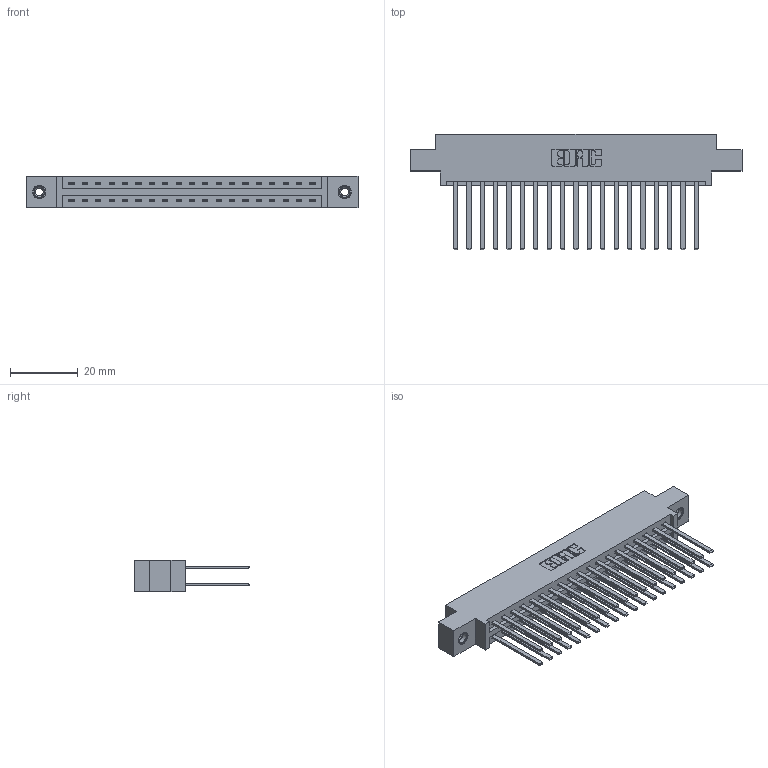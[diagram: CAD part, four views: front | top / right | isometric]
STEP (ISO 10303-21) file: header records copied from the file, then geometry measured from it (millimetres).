
FILE_DESCRIPTION (( 'STEP AP203' ), '1' );
FILE_NAME ('387-038-544-808.STEP', '2018-09-19T06:06:41', ( '' ), ( '' ), 'SwSTEP 2.0', 'SolidWorks 2016', '' );
FILE_SCHEMA (( 'CONFIG_CONTROL_DESIGN' ));
Length unit declared in the file: inch
Products named in the file (4): 387-038-544-808; 337 Part_0.170 Offset - 0.156 Dia-TI; 345-292-001_345-293-144; 345-250-001_345-250-003-102
Assembly tree (41 placements, depth 2):
  387-038-544-808
    337 Part_0.170 Offset - 0.156 Dia-TI
    345-292-001_345-293-144  x38
    345-250-001_345-250-003-102  x2
Bounding box: 98.3 x 34.3 x 9.4 mm (x, y, z)
Volume: 10461.9 mm3; surface area: 13475.7 mm2
Topology: 41 solids, 41 shells, 2002 faces, 5893 edges, 3870 vertices
Faces by surface type: plane 1398, cylinder 588, cone 12, torus 4
Entity records: 18840 total; most frequent: CARTESIAN_POINT 3173, ORIENTED_EDGE 3102, DIRECTION 2769, EDGE_CURVE 1551, LINE 1407, VECTOR 1407, VERTEX_POINT 1028, AXIS2_PLACEMENT_3D 681
